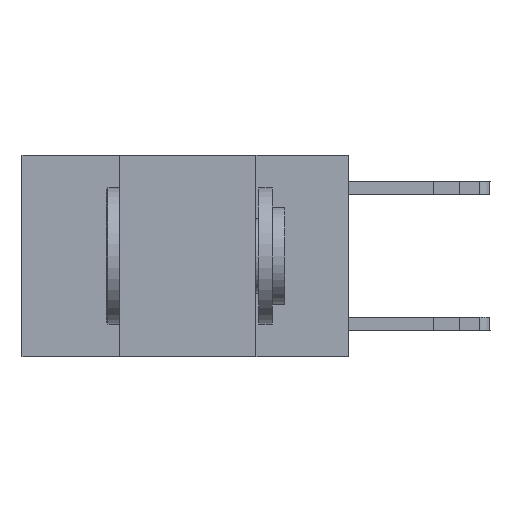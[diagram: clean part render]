
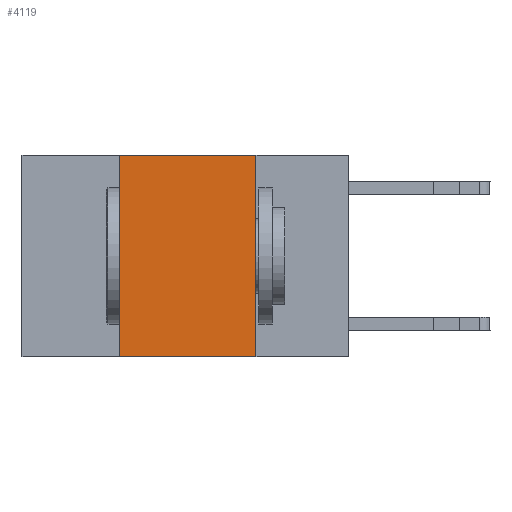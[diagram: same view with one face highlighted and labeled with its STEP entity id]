
A CAD part, left-side view. The second image highlights one B-rep face of the part: STEP entity #4119.
In plain terms, the highlighted planar face has unit normal (-1, 0, 0).
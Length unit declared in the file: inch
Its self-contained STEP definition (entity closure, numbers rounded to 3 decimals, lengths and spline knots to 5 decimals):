
#417 = CARTESIAN_POINT ( 'NONE',  ( 0., 0.42, 0. ) ) ;
#526 = CARTESIAN_POINT ( 'NONE',  ( 0., 0.17, 0. ) ) ;
#849 = VECTOR ( 'NONE', #13407, 39.37008 ) ;
#900 = DIRECTION ( 'NONE',  ( 0., 0., 1. ) ) ;
#1294 = EDGE_CURVE ( 'NONE', #27426, #13850, #2687, .T. ) ;
#1365 = ORIENTED_EDGE ( 'NONE', *, *, #10513, .T. ) ;
#1414 = CARTESIAN_POINT ( 'NONE',  ( 0., 0.6, 0. ) ) ;
#1661 = VERTEX_POINT ( 'NONE', #25392 ) ;
#2056 = AXIS2_PLACEMENT_3D ( 'NONE', #16316, #14127, #22972 ) ;
#2143 = VERTEX_POINT ( 'NONE', #417 ) ;
#2687 = LINE ( 'NONE', #526, #19317 ) ;
#4119 = ADVANCED_FACE ( 'NONE', ( #13592 ), #27440, .F. ) ;
#4413 = CARTESIAN_POINT ( 'NONE',  ( 0., 0.6, -0.37 ) ) ;
#4690 = ORIENTED_EDGE ( 'NONE', *, *, #1294, .F. ) ;
#5206 = CARTESIAN_POINT ( 'NONE',  ( 0., 0.42, 0. ) ) ;
#6564 = CARTESIAN_POINT ( 'NONE',  ( 0., 0.17, -0.37 ) ) ;
#7422 = DIRECTION ( 'NONE',  ( 0., 0., -1. ) ) ;
#9185 = VECTOR ( 'NONE', #14732, 39.37008 ) ;
#9295 = VECTOR ( 'NONE', #900, 39.37008 ) ;
#9681 = ORIENTED_EDGE ( 'NONE', *, *, #14031, .F. ) ;
#10513 = EDGE_CURVE ( 'NONE', #1661, #13850, #12831, .T. ) ;
#12831 = LINE ( 'NONE', #4413, #849 ) ;
#13407 = DIRECTION ( 'NONE',  ( 0., -1., 0. ) ) ;
#13592 = FACE_OUTER_BOUND ( 'NONE', #19437, .T. ) ;
#13850 = VERTEX_POINT ( 'NONE', #6564 ) ;
#14031 = EDGE_CURVE ( 'NONE', #1661, #2143, #20731, .T. ) ;
#14127 = DIRECTION ( 'NONE',  ( 1., 0., 0. ) ) ;
#14732 = DIRECTION ( 'NONE',  ( 0., -1., 0. ) ) ;
#15016 = LINE ( 'NONE', #1414, #9185 ) ;
#16316 = CARTESIAN_POINT ( 'NONE',  ( 0., 0.6, 0. ) ) ;
#19317 = VECTOR ( 'NONE', #7422, 39.37008 ) ;
#19437 = EDGE_LOOP ( 'NONE', ( #4690, #24524, #9681, #1365 ) ) ;
#20731 = LINE ( 'NONE', #5206, #9295 ) ;
#22972 = DIRECTION ( 'NONE',  ( 0., 0., -1. ) ) ;
#24524 = ORIENTED_EDGE ( 'NONE', *, *, #27842, .F. ) ;
#25392 = CARTESIAN_POINT ( 'NONE',  ( 0., 0.42, -0.37 ) ) ;
#27395 = CARTESIAN_POINT ( 'NONE',  ( 0., 0.17, 0. ) ) ;
#27426 = VERTEX_POINT ( 'NONE', #27395 ) ;
#27440 = PLANE ( 'NONE',  #2056 ) ;
#27842 = EDGE_CURVE ( 'NONE', #2143, #27426, #15016, .T. ) ;
